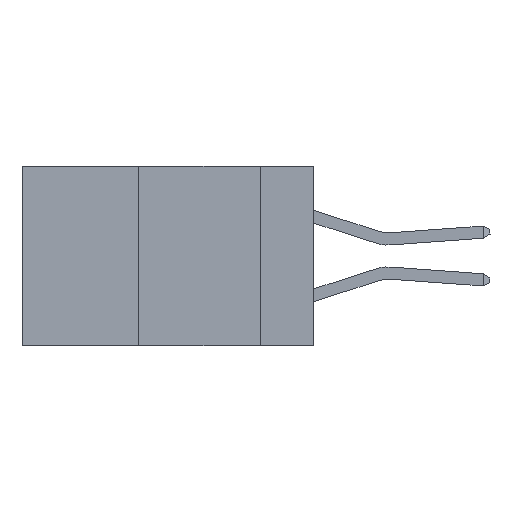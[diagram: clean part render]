
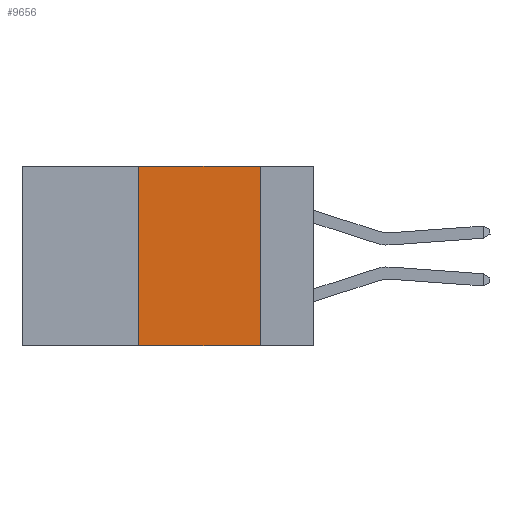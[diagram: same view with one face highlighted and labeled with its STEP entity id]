
A CAD part, left-side view. The second image highlights one B-rep face of the part: STEP entity #9656.
In plain terms, the highlighted planar face has unit normal (-1, 0, 0).
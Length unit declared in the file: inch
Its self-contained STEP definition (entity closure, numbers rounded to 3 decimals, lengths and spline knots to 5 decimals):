
#415 = EDGE_LOOP ( 'NONE', ( #3256, #13243, #4232, #2950 ) ) ;
#1277 = EDGE_CURVE ( 'NONE', #14286, #5308, #12660, .T. ) ;
#1627 = CARTESIAN_POINT ( 'NONE',  ( 0., 0.6, 0. ) ) ;
#1769 = FACE_OUTER_BOUND ( 'NONE', #415, .T. ) ;
#1863 = CARTESIAN_POINT ( 'NONE',  ( 0., 0.6, 0. ) ) ;
#2826 = PLANE ( 'NONE',  #6599 ) ;
#2895 = DIRECTION ( 'NONE',  ( 0., 0., -1. ) ) ;
#2950 = ORIENTED_EDGE ( 'NONE', *, *, #1277, .T. ) ;
#3256 = ORIENTED_EDGE ( 'NONE', *, *, #14545, .F. ) ;
#3551 = CARTESIAN_POINT ( 'NONE',  ( 0., 0.11, 0. ) ) ;
#4232 = ORIENTED_EDGE ( 'NONE', *, *, #7975, .F. ) ;
#5308 = VERTEX_POINT ( 'NONE', #11837 ) ;
#6180 = VECTOR ( 'NONE', #14193, 39.37008 ) ;
#6414 = LINE ( 'NONE', #8718, #9118 ) ;
#6599 = AXIS2_PLACEMENT_3D ( 'NONE', #1627, #13185, #2895 ) ;
#6703 = DIRECTION ( 'NONE',  ( 0., 0., 1. ) ) ;
#6825 = VERTEX_POINT ( 'NONE', #3551 ) ;
#7416 = VECTOR ( 'NONE', #10815, 39.37008 ) ;
#7742 = CARTESIAN_POINT ( 'NONE',  ( 0., 0.36, 0. ) ) ;
#7816 = DIRECTION ( 'NONE',  ( 0., 0., -1. ) ) ;
#7975 = EDGE_CURVE ( 'NONE', #14286, #11777, #13396, .T. ) ;
#8688 = CARTESIAN_POINT ( 'NONE',  ( 0., 0.36, 0. ) ) ;
#8718 = CARTESIAN_POINT ( 'NONE',  ( 0., 0.11, 0. ) ) ;
#9118 = VECTOR ( 'NONE', #7816, 39.37008 ) ;
#9314 = CARTESIAN_POINT ( 'NONE',  ( 0., 0.36, -0.37 ) ) ;
#9656 = ADVANCED_FACE ( 'NONE', ( #1769 ), #2826, .F. ) ;
#10583 = VECTOR ( 'NONE', #6703, 39.37008 ) ;
#10815 = DIRECTION ( 'NONE',  ( 0., -1., 0. ) ) ;
#11698 = CARTESIAN_POINT ( 'NONE',  ( 0., 0.6, -0.37 ) ) ;
#11777 = VERTEX_POINT ( 'NONE', #8688 ) ;
#11837 = CARTESIAN_POINT ( 'NONE',  ( 0., 0.11, -0.37 ) ) ;
#12010 = LINE ( 'NONE', #1863, #6180 ) ;
#12660 = LINE ( 'NONE', #11698, #7416 ) ;
#13185 = DIRECTION ( 'NONE',  ( 1., 0., 0. ) ) ;
#13243 = ORIENTED_EDGE ( 'NONE', *, *, #13501, .F. ) ;
#13396 = LINE ( 'NONE', #7742, #10583 ) ;
#13501 = EDGE_CURVE ( 'NONE', #11777, #6825, #12010, .T. ) ;
#14193 = DIRECTION ( 'NONE',  ( 0., -1., 0. ) ) ;
#14286 = VERTEX_POINT ( 'NONE', #9314 ) ;
#14545 = EDGE_CURVE ( 'NONE', #6825, #5308, #6414, .T. ) ;
